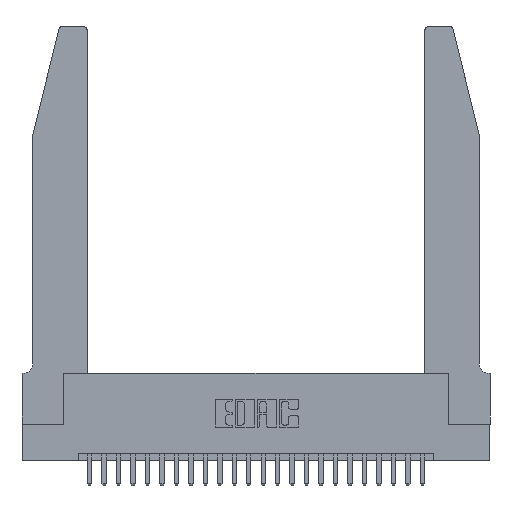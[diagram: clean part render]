
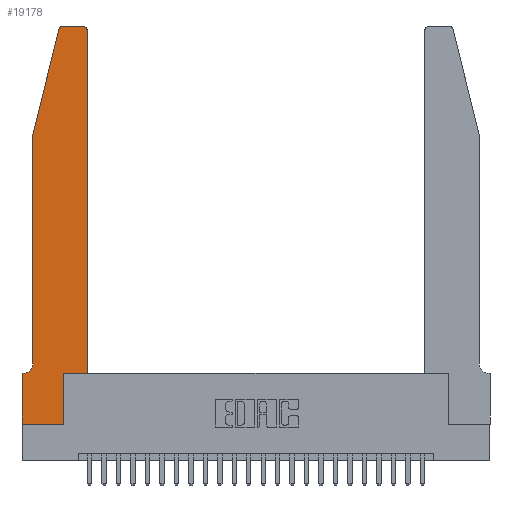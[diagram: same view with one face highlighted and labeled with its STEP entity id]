
A CAD part, top view. The second image highlights one B-rep face of the part: STEP entity #19178.
In plain terms, the highlighted planar face has unit normal (0, 0, 1).
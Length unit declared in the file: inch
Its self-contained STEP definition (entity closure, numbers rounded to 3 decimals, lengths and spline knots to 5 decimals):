
#168 = DIRECTION ( 'NONE',  ( -1., 0., 0. ) ) ;
#1085 = LINE ( 'NONE', #9493, #7461 ) ;
#1829 = CARTESIAN_POINT ( 'NONE',  ( 0.25487, 2.72718, 0.37 ) ) ;
#2029 = VERTEX_POINT ( 'NONE', #1829 ) ;
#2975 = AXIS2_PLACEMENT_3D ( 'NONE', #16744, #4571, #12377 ) ;
#3295 = VERTEX_POINT ( 'NONE', #9381 ) ;
#3931 = ORIENTED_EDGE ( 'NONE', *, *, #10944, .T. ) ;
#3958 = ORIENTED_EDGE ( 'NONE', *, *, #13699, .T. ) ;
#4361 = CARTESIAN_POINT ( 'NONE',  ( 0., 0., 0.37 ) ) ;
#4487 = ORIENTED_EDGE ( 'NONE', *, *, #19012, .T. ) ;
#4571 = DIRECTION ( 'NONE',  ( 0., 0., 1. ) ) ;
#4782 = CARTESIAN_POINT ( 'NONE',  ( 0., 0., 0.37 ) ) ;
#5413 = DIRECTION ( 'NONE',  ( 1., 0., 0. ) ) ;
#5460 = VERTEX_POINT ( 'NONE', #17961 ) ;
#5589 = VERTEX_POINT ( 'NONE', #24846 ) ;
#5904 = CIRCLE ( 'NONE', #6334, 0.07 ) ;
#5956 = CARTESIAN_POINT ( 'NONE',  ( 0.0055, 0.35, 0.37 ) ) ;
#5998 = LINE ( 'NONE', #19470, #21840 ) ;
#6325 = VECTOR ( 'NONE', #21422, 39.37008 ) ;
#6334 = AXIS2_PLACEMENT_3D ( 'NONE', #12119, #24119, #26140 ) ;
#6800 = ORIENTED_EDGE ( 'NONE', *, *, #18941, .T. ) ;
#7213 = EDGE_CURVE ( 'NONE', #19739, #23263, #19292, .T. ) ;
#7461 = VECTOR ( 'NONE', #15398, 39.37008 ) ;
#7641 = LINE ( 'NONE', #21191, #11065 ) ;
#8274 = CARTESIAN_POINT ( 'NONE',  ( 0.2605, 2.75, 0.37 ) ) ;
#8442 = ORIENTED_EDGE ( 'NONE', *, *, #22850, .T. ) ;
#9381 = CARTESIAN_POINT ( 'NONE',  ( 0.2865, 0.35, 0.37 ) ) ;
#9493 = CARTESIAN_POINT ( 'NONE',  ( 0.0755, 0.35, 0.37 ) ) ;
#9627 = ORIENTED_EDGE ( 'NONE', *, *, #23742, .T. ) ;
#9704 = EDGE_CURVE ( 'NONE', #21290, #2029, #18868, .T. ) ;
#10532 = DIRECTION ( 'NONE',  ( 0., 0., 1. ) ) ;
#10552 = CARTESIAN_POINT ( 'NONE',  ( 0.0755, 0.42, 0.37 ) ) ;
#10714 = CARTESIAN_POINT ( 'NONE',  ( 0.4505, 2.72, 0.37 ) ) ;
#10944 = EDGE_CURVE ( 'NONE', #5460, #23255, #20374, .T. ) ;
#11065 = VECTOR ( 'NONE', #23228, 39.37008 ) ;
#11238 = EDGE_LOOP ( 'NONE', ( #6800, #18070, #9627, #8442, #4487, #11564, #3958, #19199, #14682, #12206, #3931, #14544 ) ) ;
#11564 = ORIENTED_EDGE ( 'NONE', *, *, #20506, .T. ) ;
#12119 = CARTESIAN_POINT ( 'NONE',  ( 0.0055, 0.42, 0.37 ) ) ;
#12131 = VERTEX_POINT ( 'NONE', #5956 ) ;
#12132 = AXIS2_PLACEMENT_3D ( 'NONE', #20282, #24413, #26099 ) ;
#12206 = ORIENTED_EDGE ( 'NONE', *, *, #23053, .T. ) ;
#12377 = DIRECTION ( 'NONE',  ( 1., 0., 0. ) ) ;
#12783 = DIRECTION ( 'NONE',  ( 1., 0., 0. ) ) ;
#13069 = CARTESIAN_POINT ( 'NONE',  ( 0.4505, 0.35, 0.37 ) ) ;
#13565 = CIRCLE ( 'NONE', #12132, 0.03 ) ;
#13699 = EDGE_CURVE ( 'NONE', #24036, #19739, #15878, .T. ) ;
#13833 = CARTESIAN_POINT ( 'NONE',  ( 0.284, 2.75, 0.37 ) ) ;
#14121 = CARTESIAN_POINT ( 'NONE',  ( 0., 0.35, 0.37 ) ) ;
#14281 = DIRECTION ( 'NONE',  ( 0., -1., 0. ) ) ;
#14544 = ORIENTED_EDGE ( 'NONE', *, *, #24016, .T. ) ;
#14652 = VERTEX_POINT ( 'NONE', #10552 ) ;
#14682 = ORIENTED_EDGE ( 'NONE', *, *, #24513, .T. ) ;
#14963 = VECTOR ( 'NONE', #23283, 39.37008 ) ;
#15047 = FACE_OUTER_BOUND ( 'NONE', #11238, .T. ) ;
#15398 = DIRECTION ( 'NONE',  ( -1., 0., 0. ) ) ;
#15878 = LINE ( 'NONE', #24360, #20992 ) ;
#16677 = LINE ( 'NONE', #19923, #18257 ) ;
#16744 = CARTESIAN_POINT ( 'NONE',  ( 0., 0.35, 0.37 ) ) ;
#17961 = CARTESIAN_POINT ( 'NONE',  ( 0.4505, 0.35, 0.37 ) ) ;
#18070 = ORIENTED_EDGE ( 'NONE', *, *, #9704, .T. ) ;
#18257 = VECTOR ( 'NONE', #21780, 39.37008 ) ;
#18584 = CARTESIAN_POINT ( 'NONE',  ( 0.2865, 0., 0.37 ) ) ;
#18868 = CIRCLE ( 'NONE', #22114, 0.03 ) ;
#18941 = EDGE_CURVE ( 'NONE', #5589, #21290, #25196, .T. ) ;
#19012 = EDGE_CURVE ( 'NONE', #14652, #12131, #5904, .T. ) ;
#19054 = DIRECTION ( 'NONE',  ( 1., 0., 0. ) ) ;
#19178 = ADVANCED_FACE ( 'NONE', ( #15047 ), #22778, .T. ) ;
#19199 = ORIENTED_EDGE ( 'NONE', *, *, #7213, .T. ) ;
#19292 = LINE ( 'NONE', #4782, #19612 ) ;
#19307 = LINE ( 'NONE', #23280, #6325 ) ;
#19470 = CARTESIAN_POINT ( 'NONE',  ( 0.4505, 0.35, 0.37 ) ) ;
#19612 = VECTOR ( 'NONE', #12783, 39.37008 ) ;
#19739 = VERTEX_POINT ( 'NONE', #4361 ) ;
#19857 = VERTEX_POINT ( 'NONE', #22937 ) ;
#19923 = CARTESIAN_POINT ( 'NONE',  ( 0.2865, 0.35, 0.37 ) ) ;
#20282 = CARTESIAN_POINT ( 'NONE',  ( 0.4205, 2.72, 0.37 ) ) ;
#20374 = LINE ( 'NONE', #13069, #14963 ) ;
#20506 = EDGE_CURVE ( 'NONE', #12131, #24036, #1085, .T. ) ;
#20651 = CARTESIAN_POINT ( 'NONE',  ( 0.284, 2.72, 0.37 ) ) ;
#20992 = VECTOR ( 'NONE', #14281, 39.37008 ) ;
#21191 = CARTESIAN_POINT ( 'NONE',  ( 0.0755, 2., 0.37 ) ) ;
#21290 = VERTEX_POINT ( 'NONE', #13833 ) ;
#21422 = DIRECTION ( 'NONE',  ( 0., -1., 0. ) ) ;
#21780 = DIRECTION ( 'NONE',  ( 0., 1., 0. ) ) ;
#21840 = VECTOR ( 'NONE', #5413, 39.37008 ) ;
#22114 = AXIS2_PLACEMENT_3D ( 'NONE', #20651, #10532, #19054 ) ;
#22778 = PLANE ( 'NONE',  #2975 ) ;
#22850 = EDGE_CURVE ( 'NONE', #19857, #14652, #19307, .T. ) ;
#22937 = CARTESIAN_POINT ( 'NONE',  ( 0.0755, 2., 0.37 ) ) ;
#23053 = EDGE_CURVE ( 'NONE', #3295, #5460, #5998, .T. ) ;
#23228 = DIRECTION ( 'NONE',  ( -0.239, -0.971, 0. ) ) ;
#23255 = VERTEX_POINT ( 'NONE', #10714 ) ;
#23263 = VERTEX_POINT ( 'NONE', #18584 ) ;
#23280 = CARTESIAN_POINT ( 'NONE',  ( 0.0755, 2., 0.37 ) ) ;
#23283 = DIRECTION ( 'NONE',  ( 0., 1., 0. ) ) ;
#23742 = EDGE_CURVE ( 'NONE', #2029, #19857, #7641, .T. ) ;
#24016 = EDGE_CURVE ( 'NONE', #23255, #5589, #13565, .T. ) ;
#24036 = VERTEX_POINT ( 'NONE', #14121 ) ;
#24119 = DIRECTION ( 'NONE',  ( 0., 0., -1. ) ) ;
#24260 = VECTOR ( 'NONE', #168, 39.37008 ) ;
#24360 = CARTESIAN_POINT ( 'NONE',  ( 0., 0., 0.37 ) ) ;
#24413 = DIRECTION ( 'NONE',  ( 0., 0., 1. ) ) ;
#24513 = EDGE_CURVE ( 'NONE', #23263, #3295, #16677, .T. ) ;
#24846 = CARTESIAN_POINT ( 'NONE',  ( 0.4205, 2.75, 0.37 ) ) ;
#25196 = LINE ( 'NONE', #8274, #24260 ) ;
#26099 = DIRECTION ( 'NONE',  ( 1., 0., 0. ) ) ;
#26140 = DIRECTION ( 'NONE',  ( -1., 0., 0. ) ) ;
